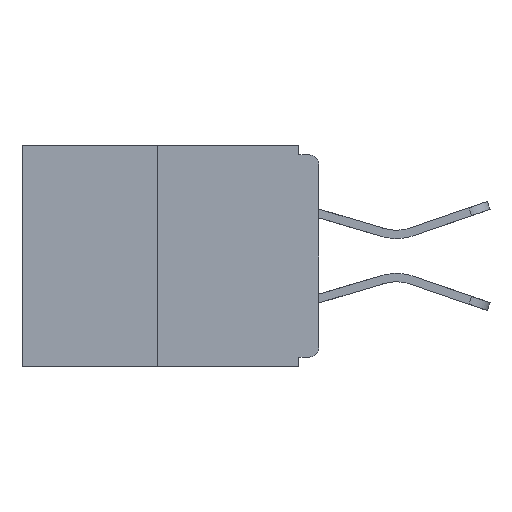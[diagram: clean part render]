
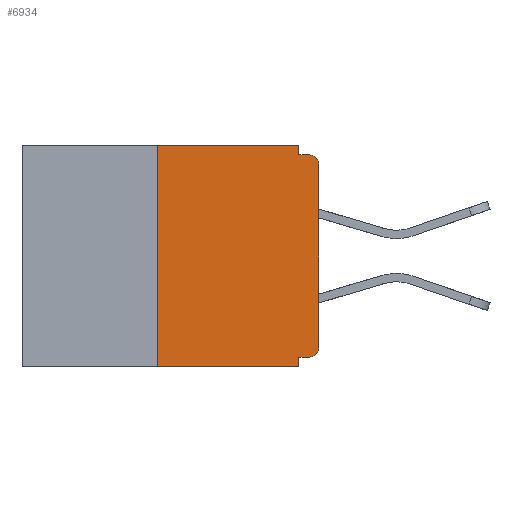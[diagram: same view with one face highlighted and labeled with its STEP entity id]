
A CAD part, left-side view. The second image highlights one B-rep face of the part: STEP entity #6934.
In plain terms, the highlighted planar face has unit normal (-1, 0, 0).
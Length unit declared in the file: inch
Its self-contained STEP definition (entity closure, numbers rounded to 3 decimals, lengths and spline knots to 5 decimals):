
#332 = CARTESIAN_POINT ( 'NONE',  ( 0., 0., -0.328 ) ) ;
#573 = CARTESIAN_POINT ( 'NONE',  ( 0., 0.031, -0.343 ) ) ;
#966 = VERTEX_POINT ( 'NONE', #5923 ) ;
#975 = LINE ( 'NONE', #3677, #13980 ) ;
#1058 = DIRECTION ( 'NONE',  ( 0., 0., 1. ) ) ;
#1149 = EDGE_CURVE ( 'NONE', #11704, #12278, #6132, .T. ) ;
#1508 = CARTESIAN_POINT ( 'NONE',  ( 0., 0.46, 0. ) ) ;
#1583 = DIRECTION ( 'NONE',  ( 0., -1., 0. ) ) ;
#1670 = LINE ( 'NONE', #13183, #6011 ) ;
#1886 = CARTESIAN_POINT ( 'NONE',  ( 0., 0.015, -0.313 ) ) ;
#1997 = EDGE_CURVE ( 'NONE', #7188, #2779, #7019, .T. ) ;
#2062 = CARTESIAN_POINT ( 'NONE',  ( 0., 0.015, -0.015 ) ) ;
#2155 = VECTOR ( 'NONE', #3479, 39.37008 ) ;
#2576 = VECTOR ( 'NONE', #1058, 39.37008 ) ;
#2606 = AXIS2_PLACEMENT_3D ( 'NONE', #1508, #8019, #6928 ) ;
#2779 = VERTEX_POINT ( 'NONE', #2062 ) ;
#2842 = DIRECTION ( 'NONE',  ( -1., 0., 0. ) ) ;
#2872 = ORIENTED_EDGE ( 'NONE', *, *, #12475, .F. ) ;
#2996 = LINE ( 'NONE', #332, #2155 ) ;
#3082 = ORIENTED_EDGE ( 'NONE', *, *, #11042, .F. ) ;
#3135 = DIRECTION ( 'NONE',  ( 0., 0., -1. ) ) ;
#3333 = CARTESIAN_POINT ( 'NONE',  ( 0., 0.031, 0. ) ) ;
#3479 = DIRECTION ( 'NONE',  ( 0., 1., 0. ) ) ;
#3553 = DIRECTION ( 'NONE',  ( 0., 0., 1. ) ) ;
#3677 = CARTESIAN_POINT ( 'NONE',  ( 0., 0.031, -0.343 ) ) ;
#4009 = EDGE_CURVE ( 'NONE', #10485, #8873, #7633, .T. ) ;
#4424 = CARTESIAN_POINT ( 'NONE',  ( 0., 0., -0.015 ) ) ;
#4434 = EDGE_LOOP ( 'NONE', ( #3082, #2872, #5433, #12002, #11738, #8635, #10438, #10699, #13502, #12397 ) ) ;
#4531 = CARTESIAN_POINT ( 'NONE',  ( 0., 0., -0.03 ) ) ;
#4768 = CARTESIAN_POINT ( 'NONE',  ( 0., 0., 0. ) ) ;
#4772 = VERTEX_POINT ( 'NONE', #3333 ) ;
#5126 = EDGE_CURVE ( 'NONE', #4772, #11839, #1670, .T. ) ;
#5133 = DIRECTION ( 'NONE',  ( 0., -1., 0. ) ) ;
#5433 = ORIENTED_EDGE ( 'NONE', *, *, #4009, .T. ) ;
#5548 = LINE ( 'NONE', #4768, #2576 ) ;
#5636 = AXIS2_PLACEMENT_3D ( 'NONE', #11572, #2842, #10574 ) ;
#5828 = PLANE ( 'NONE',  #2606 ) ;
#5868 = DIRECTION ( 'NONE',  ( 0., 0., -1. ) ) ;
#5923 = CARTESIAN_POINT ( 'NONE',  ( 0., 0.25, 0. ) ) ;
#5924 = CARTESIAN_POINT ( 'NONE',  ( 0., 0.25, 0. ) ) ;
#6011 = VECTOR ( 'NONE', #3135, 39.37008 ) ;
#6127 = FACE_OUTER_BOUND ( 'NONE', #4434, .T. ) ;
#6132 = CIRCLE ( 'NONE', #10466, 0.015 ) ;
#6598 = EDGE_CURVE ( 'NONE', #11704, #12816, #2996, .T. ) ;
#6894 = VECTOR ( 'NONE', #5133, 39.37008 ) ;
#6928 = DIRECTION ( 'NONE',  ( 0., 0., -1. ) ) ;
#6934 = ADVANCED_FACE ( 'NONE', ( #6127 ), #5828, .F. ) ;
#7019 = CIRCLE ( 'NONE', #5636, 0.015 ) ;
#7188 = VERTEX_POINT ( 'NONE', #4531 ) ;
#7448 = EDGE_CURVE ( 'NONE', #11839, #2779, #9412, .T. ) ;
#7526 = CARTESIAN_POINT ( 'NONE',  ( 0., 0.031, -0.015 ) ) ;
#7633 = LINE ( 'NONE', #10279, #8819 ) ;
#8019 = DIRECTION ( 'NONE',  ( 1., 0., 0. ) ) ;
#8635 = ORIENTED_EDGE ( 'NONE', *, *, #1149, .T. ) ;
#8819 = VECTOR ( 'NONE', #1583, 39.37008 ) ;
#8873 = VERTEX_POINT ( 'NONE', #573 ) ;
#9041 = LINE ( 'NONE', #5924, #11461 ) ;
#9182 = EDGE_CURVE ( 'NONE', #12278, #7188, #5548, .T. ) ;
#9412 = LINE ( 'NONE', #4424, #10462 ) ;
#9666 = DIRECTION ( 'NONE',  ( -1., 0., 0. ) ) ;
#9825 = LINE ( 'NONE', #10489, #6894 ) ;
#10106 = CARTESIAN_POINT ( 'NONE',  ( 0., 0.031, -0.328 ) ) ;
#10123 = CARTESIAN_POINT ( 'NONE',  ( 0., 0., -0.313 ) ) ;
#10279 = CARTESIAN_POINT ( 'NONE',  ( 0., 0.46, -0.343 ) ) ;
#10438 = ORIENTED_EDGE ( 'NONE', *, *, #9182, .T. ) ;
#10462 = VECTOR ( 'NONE', #13294, 39.37008 ) ;
#10466 = AXIS2_PLACEMENT_3D ( 'NONE', #1886, #9666, #11689 ) ;
#10485 = VERTEX_POINT ( 'NONE', #12958 ) ;
#10489 = CARTESIAN_POINT ( 'NONE',  ( 0., 0.46, 0. ) ) ;
#10526 = CARTESIAN_POINT ( 'NONE',  ( 0., 0.015, -0.328 ) ) ;
#10574 = DIRECTION ( 'NONE',  ( 0., 0., -1. ) ) ;
#10699 = ORIENTED_EDGE ( 'NONE', *, *, #1997, .T. ) ;
#10891 = EDGE_CURVE ( 'NONE', #12816, #8873, #975, .T. ) ;
#11042 = EDGE_CURVE ( 'NONE', #966, #4772, #9825, .T. ) ;
#11461 = VECTOR ( 'NONE', #3553, 39.37008 ) ;
#11572 = CARTESIAN_POINT ( 'NONE',  ( 0., 0.015, -0.03 ) ) ;
#11689 = DIRECTION ( 'NONE',  ( 0., 0., -1. ) ) ;
#11704 = VERTEX_POINT ( 'NONE', #10526 ) ;
#11738 = ORIENTED_EDGE ( 'NONE', *, *, #6598, .F. ) ;
#11839 = VERTEX_POINT ( 'NONE', #7526 ) ;
#12002 = ORIENTED_EDGE ( 'NONE', *, *, #10891, .F. ) ;
#12278 = VERTEX_POINT ( 'NONE', #10123 ) ;
#12397 = ORIENTED_EDGE ( 'NONE', *, *, #5126, .F. ) ;
#12475 = EDGE_CURVE ( 'NONE', #10485, #966, #9041, .T. ) ;
#12816 = VERTEX_POINT ( 'NONE', #10106 ) ;
#12958 = CARTESIAN_POINT ( 'NONE',  ( 0., 0.25, -0.343 ) ) ;
#13183 = CARTESIAN_POINT ( 'NONE',  ( 0., 0.031, 0. ) ) ;
#13294 = DIRECTION ( 'NONE',  ( 0., -1., 0. ) ) ;
#13502 = ORIENTED_EDGE ( 'NONE', *, *, #7448, .F. ) ;
#13980 = VECTOR ( 'NONE', #5868, 39.37008 ) ;
